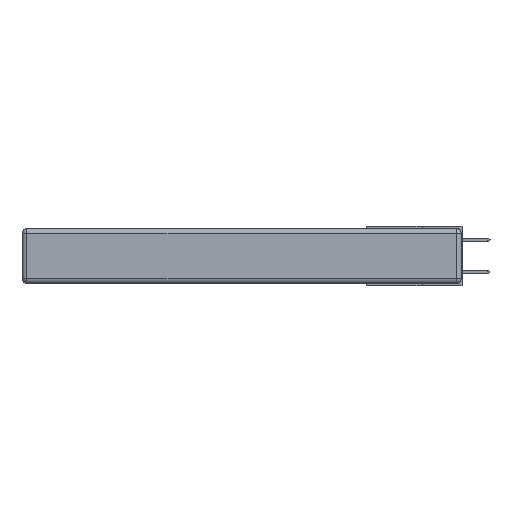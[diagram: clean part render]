
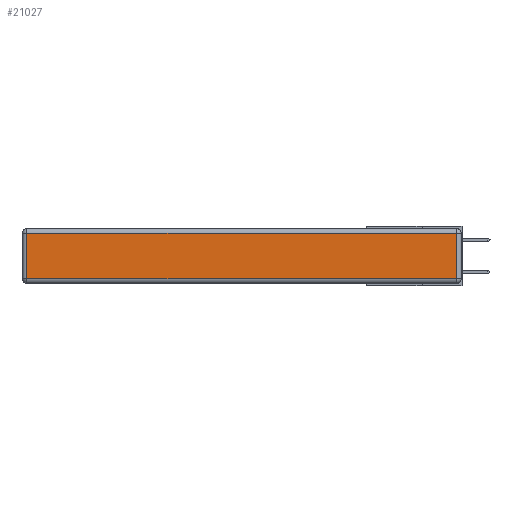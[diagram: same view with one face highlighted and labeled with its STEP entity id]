
A CAD part, left-side view. The second image highlights one B-rep face of the part: STEP entity #21027.
In plain terms, the highlighted planar face has unit normal (-1, 0, 0).
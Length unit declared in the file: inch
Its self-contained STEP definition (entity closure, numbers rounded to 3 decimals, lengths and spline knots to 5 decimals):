
#1291 = CARTESIAN_POINT ( 'NONE',  ( 0., 0., -0.343 ) ) ;
#3498 = DIRECTION ( 'NONE',  ( 0., 0., 1. ) ) ;
#3796 = PLANE ( 'NONE',  #11235 ) ;
#3907 = DIRECTION ( 'NONE',  ( -1., 0., 0. ) ) ;
#4284 = LINE ( 'NONE', #17038, #27391 ) ;
#4614 = FACE_OUTER_BOUND ( 'NONE', #16606, .T. ) ;
#7506 = ORIENTED_EDGE ( 'NONE', *, *, #9880, .T. ) ;
#8572 = CARTESIAN_POINT ( 'NONE',  ( 0., 2.72, -0.03 ) ) ;
#9477 = LINE ( 'NONE', #21308, #19130 ) ;
#9482 = VECTOR ( 'NONE', #24384, 39.37008 ) ;
#9880 = EDGE_CURVE ( 'NONE', #28301, #14432, #19796, .T. ) ;
#11235 = AXIS2_PLACEMENT_3D ( 'NONE', #1291, #3907, #20654 ) ;
#12768 = ORIENTED_EDGE ( 'NONE', *, *, #20547, .T. ) ;
#12909 = CARTESIAN_POINT ( 'NONE',  ( 0., 0.03, -0.03 ) ) ;
#13115 = EDGE_CURVE ( 'NONE', #22291, #16190, #21351, .T. ) ;
#13504 = VECTOR ( 'NONE', #3498, 39.37008 ) ;
#13571 = ORIENTED_EDGE ( 'NONE', *, *, #30262, .T. ) ;
#14432 = VERTEX_POINT ( 'NONE', #12909 ) ;
#14814 = CARTESIAN_POINT ( 'NONE',  ( 0., 0.03, -0.313 ) ) ;
#16190 = VERTEX_POINT ( 'NONE', #24754 ) ;
#16606 = EDGE_LOOP ( 'NONE', ( #12768, #7506, #13571, #22556 ) ) ;
#17038 = CARTESIAN_POINT ( 'NONE',  ( 0., 0., -0.313 ) ) ;
#18623 = DIRECTION ( 'NONE',  ( 0., 1., 0. ) ) ;
#19130 = VECTOR ( 'NONE', #18623, 39.37008 ) ;
#19537 = DIRECTION ( 'NONE',  ( 0., -1., 0. ) ) ;
#19796 = LINE ( 'NONE', #27159, #13504 ) ;
#20547 = EDGE_CURVE ( 'NONE', #16190, #28301, #4284, .T. ) ;
#20654 = DIRECTION ( 'NONE',  ( 0., 0., 1. ) ) ;
#21027 = ADVANCED_FACE ( 'NONE', ( #4614 ), #3796, .T. ) ;
#21308 = CARTESIAN_POINT ( 'NONE',  ( 0., 2.75, -0.03 ) ) ;
#21351 = LINE ( 'NONE', #23612, #9482 ) ;
#22291 = VERTEX_POINT ( 'NONE', #8572 ) ;
#22556 = ORIENTED_EDGE ( 'NONE', *, *, #13115, .T. ) ;
#23612 = CARTESIAN_POINT ( 'NONE',  ( 0., 2.72, -0.343 ) ) ;
#24384 = DIRECTION ( 'NONE',  ( 0., 0., -1. ) ) ;
#24754 = CARTESIAN_POINT ( 'NONE',  ( 0., 2.72, -0.313 ) ) ;
#27159 = CARTESIAN_POINT ( 'NONE',  ( 0., 0.03, -0.343 ) ) ;
#27391 = VECTOR ( 'NONE', #19537, 39.37008 ) ;
#28301 = VERTEX_POINT ( 'NONE', #14814 ) ;
#30262 = EDGE_CURVE ( 'NONE', #14432, #22291, #9477, .T. ) ;
